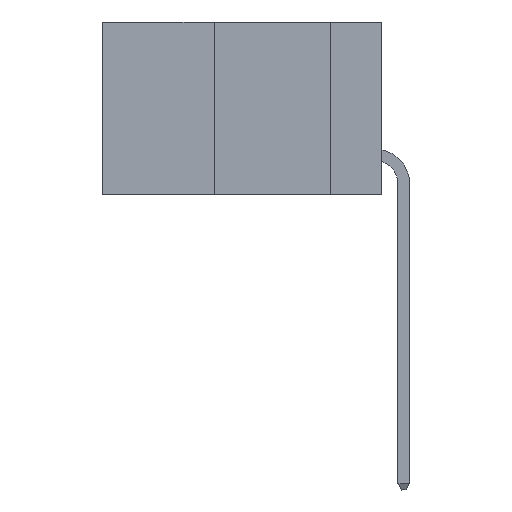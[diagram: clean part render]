
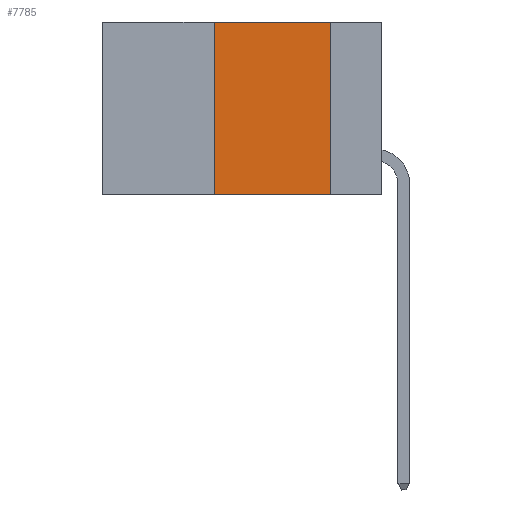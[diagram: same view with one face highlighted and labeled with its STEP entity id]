
A CAD part, left-side view. The second image highlights one B-rep face of the part: STEP entity #7785.
In plain terms, the highlighted planar face has unit normal (-1, 0, 0).
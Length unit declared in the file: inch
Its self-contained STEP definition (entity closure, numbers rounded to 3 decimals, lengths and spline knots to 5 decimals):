
#36 = EDGE_CURVE ( 'NONE', #15648, #10535, #2374, .T. ) ;
#1248 = CARTESIAN_POINT ( 'NONE',  ( 0., 0.36, -0.37 ) ) ;
#2074 = PLANE ( 'NONE',  #13688 ) ;
#2129 = DIRECTION ( 'NONE',  ( 1., 0., 0. ) ) ;
#2374 = LINE ( 'NONE', #13581, #9437 ) ;
#3280 = VERTEX_POINT ( 'NONE', #1248 ) ;
#3371 = ORIENTED_EDGE ( 'NONE', *, *, #9340, .T. ) ;
#3608 = CARTESIAN_POINT ( 'NONE',  ( 0., 0.36, 0. ) ) ;
#4476 = DIRECTION ( 'NONE',  ( 0., -1., 0. ) ) ;
#4788 = ORIENTED_EDGE ( 'NONE', *, *, #36, .F. ) ;
#4990 = LINE ( 'NONE', #8649, #11538 ) ;
#5861 = LINE ( 'NONE', #3608, #6951 ) ;
#6439 = CARTESIAN_POINT ( 'NONE',  ( 0., 0.11, 0. ) ) ;
#6585 = DIRECTION ( 'NONE',  ( 0., 0., -1. ) ) ;
#6951 = VECTOR ( 'NONE', #9263, 39.37008 ) ;
#7051 = DIRECTION ( 'NONE',  ( 0., -1., 0. ) ) ;
#7785 = ADVANCED_FACE ( 'NONE', ( #14280 ), #2074, .F. ) ;
#7878 = DIRECTION ( 'NONE',  ( 0., 0., -1. ) ) ;
#8070 = VECTOR ( 'NONE', #7051, 39.37008 ) ;
#8649 = CARTESIAN_POINT ( 'NONE',  ( 0., 0.6, -0.37 ) ) ;
#9202 = EDGE_CURVE ( 'NONE', #3280, #16317, #5861, .T. ) ;
#9263 = DIRECTION ( 'NONE',  ( 0., 0., 1. ) ) ;
#9288 = EDGE_CURVE ( 'NONE', #16317, #15648, #18151, .T. ) ;
#9340 = EDGE_CURVE ( 'NONE', #3280, #10535, #4990, .T. ) ;
#9437 = VECTOR ( 'NONE', #6585, 39.37008 ) ;
#10349 = CARTESIAN_POINT ( 'NONE',  ( 0., 0.11, -0.37 ) ) ;
#10535 = VERTEX_POINT ( 'NONE', #10349 ) ;
#11538 = VECTOR ( 'NONE', #4476, 39.37008 ) ;
#11897 = EDGE_LOOP ( 'NONE', ( #4788, #17481, #18136, #3371 ) ) ;
#13581 = CARTESIAN_POINT ( 'NONE',  ( 0., 0.11, 0. ) ) ;
#13688 = AXIS2_PLACEMENT_3D ( 'NONE', #17563, #2129, #7878 ) ;
#14280 = FACE_OUTER_BOUND ( 'NONE', #11897, .T. ) ;
#15648 = VERTEX_POINT ( 'NONE', #6439 ) ;
#16317 = VERTEX_POINT ( 'NONE', #16465 ) ;
#16465 = CARTESIAN_POINT ( 'NONE',  ( 0., 0.36, 0. ) ) ;
#17481 = ORIENTED_EDGE ( 'NONE', *, *, #9288, .F. ) ;
#17502 = CARTESIAN_POINT ( 'NONE',  ( 0., 0.6, 0. ) ) ;
#17563 = CARTESIAN_POINT ( 'NONE',  ( 0., 0.6, 0. ) ) ;
#18136 = ORIENTED_EDGE ( 'NONE', *, *, #9202, .F. ) ;
#18151 = LINE ( 'NONE', #17502, #8070 ) ;
